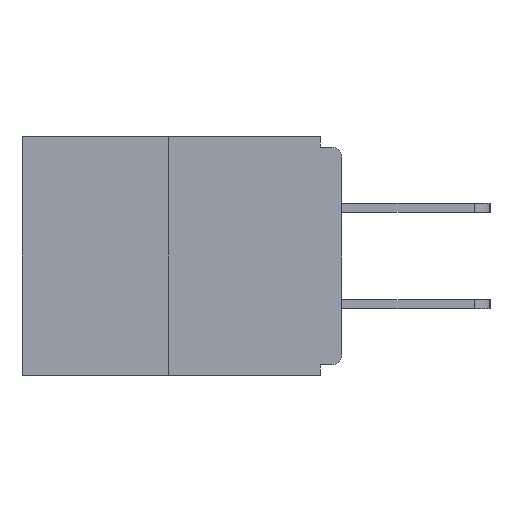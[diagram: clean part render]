
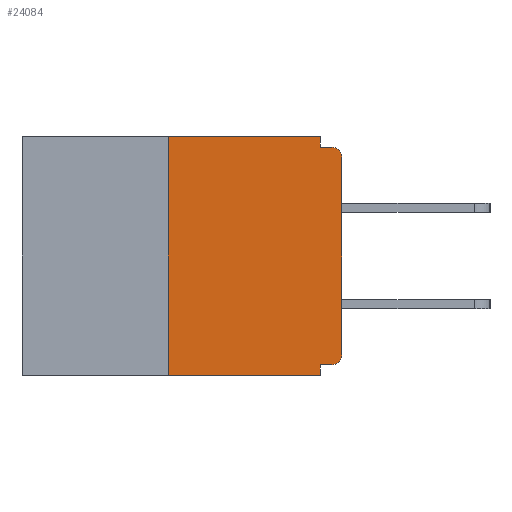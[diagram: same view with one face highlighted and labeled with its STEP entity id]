
A CAD part, left-side view. The second image highlights one B-rep face of the part: STEP entity #24084.
In plain terms, the highlighted planar face has unit normal (-1, 0, 0).
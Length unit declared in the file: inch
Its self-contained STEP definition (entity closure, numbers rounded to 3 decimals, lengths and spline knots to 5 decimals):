
#479 = CARTESIAN_POINT ( 'NONE',  ( 0., 0., -0.015 ) ) ;
#733 = ORIENTED_EDGE ( 'NONE', *, *, #24782, .F. ) ;
#1208 = VERTEX_POINT ( 'NONE', #2140 ) ;
#2140 = CARTESIAN_POINT ( 'NONE',  ( 0., 0.25, -0.343 ) ) ;
#2217 = VERTEX_POINT ( 'NONE', #22317 ) ;
#2232 = CARTESIAN_POINT ( 'NONE',  ( 0., 0., 0. ) ) ;
#2408 = DIRECTION ( 'NONE',  ( 0., 0., -1. ) ) ;
#2773 = CARTESIAN_POINT ( 'NONE',  ( 0., 0.46, 0. ) ) ;
#3001 = DIRECTION ( 'NONE',  ( 0., -1., 0. ) ) ;
#3303 = EDGE_CURVE ( 'NONE', #14553, #17531, #26968, .T. ) ;
#3306 = VERTEX_POINT ( 'NONE', #26632 ) ;
#3439 = VECTOR ( 'NONE', #9240, 39.37008 ) ;
#4180 = AXIS2_PLACEMENT_3D ( 'NONE', #10762, #8882, #2408 ) ;
#5092 = DIRECTION ( 'NONE',  ( 0., -1., 0. ) ) ;
#5288 = CARTESIAN_POINT ( 'NONE',  ( 0., 0., -0.03 ) ) ;
#5562 = ORIENTED_EDGE ( 'NONE', *, *, #7848, .T. ) ;
#6050 = ORIENTED_EDGE ( 'NONE', *, *, #3303, .T. ) ;
#6317 = ORIENTED_EDGE ( 'NONE', *, *, #28111, .F. ) ;
#7618 = LINE ( 'NONE', #24340, #26913 ) ;
#7848 = EDGE_CURVE ( 'NONE', #1208, #15797, #12713, .T. ) ;
#7966 = VERTEX_POINT ( 'NONE', #12307 ) ;
#8200 = DIRECTION ( 'NONE',  ( 0., 0., -1. ) ) ;
#8882 = DIRECTION ( 'NONE',  ( -1., 0., 0. ) ) ;
#9086 = DIRECTION ( 'NONE',  ( 0., 0., 1. ) ) ;
#9240 = DIRECTION ( 'NONE',  ( 0., 1., 0. ) ) ;
#9381 = LINE ( 'NONE', #25007, #3439 ) ;
#9680 = ORIENTED_EDGE ( 'NONE', *, *, #12728, .F. ) ;
#9987 = DIRECTION ( 'NONE',  ( 0., 0., 1. ) ) ;
#10334 = VERTEX_POINT ( 'NONE', #25268 ) ;
#10539 = AXIS2_PLACEMENT_3D ( 'NONE', #26731, #24196, #24578 ) ;
#10762 = CARTESIAN_POINT ( 'NONE',  ( 0., 0.015, -0.313 ) ) ;
#11080 = VERTEX_POINT ( 'NONE', #20988 ) ;
#11136 = VERTEX_POINT ( 'NONE', #15093 ) ;
#11830 = EDGE_CURVE ( 'NONE', #3306, #15797, #7618, .T. ) ;
#12169 = CARTESIAN_POINT ( 'NONE',  ( 0., 0.031, -0.343 ) ) ;
#12170 = VECTOR ( 'NONE', #14246, 39.37008 ) ;
#12307 = CARTESIAN_POINT ( 'NONE',  ( 0., 0.015, -0.328 ) ) ;
#12713 = LINE ( 'NONE', #25426, #21803 ) ;
#12716 = PLANE ( 'NONE',  #27837 ) ;
#12728 = EDGE_CURVE ( 'NONE', #11136, #17531, #20529, .T. ) ;
#13058 = ORIENTED_EDGE ( 'NONE', *, *, #28562, .F. ) ;
#14246 = DIRECTION ( 'NONE',  ( 0., -1., 0. ) ) ;
#14265 = EDGE_CURVE ( 'NONE', #10334, #14553, #19406, .T. ) ;
#14553 = VERTEX_POINT ( 'NONE', #5288 ) ;
#14580 = VECTOR ( 'NONE', #5092, 39.37008 ) ;
#14859 = CARTESIAN_POINT ( 'NONE',  ( 0., 0.031, 0. ) ) ;
#14951 = EDGE_CURVE ( 'NONE', #7966, #10334, #27060, .T. ) ;
#15093 = CARTESIAN_POINT ( 'NONE',  ( 0., 0.031, -0.015 ) ) ;
#15196 = EDGE_LOOP ( 'NONE', ( #13058, #733, #5562, #18835, #19710, #15767, #25383, #6050, #9680, #6317 ) ) ;
#15767 = ORIENTED_EDGE ( 'NONE', *, *, #14951, .T. ) ;
#15797 = VERTEX_POINT ( 'NONE', #12169 ) ;
#16951 = CARTESIAN_POINT ( 'NONE',  ( 0., 0.46, 0. ) ) ;
#17133 = DIRECTION ( 'NONE',  ( 0., 0., -1. ) ) ;
#17531 = VERTEX_POINT ( 'NONE', #27202 ) ;
#18835 = ORIENTED_EDGE ( 'NONE', *, *, #11830, .F. ) ;
#19326 = EDGE_CURVE ( 'NONE', #7966, #3306, #9381, .T. ) ;
#19406 = LINE ( 'NONE', #2232, #21489 ) ;
#19710 = ORIENTED_EDGE ( 'NONE', *, *, #19326, .F. ) ;
#20522 = VECTOR ( 'NONE', #9987, 39.37008 ) ;
#20529 = LINE ( 'NONE', #479, #14580 ) ;
#20988 = CARTESIAN_POINT ( 'NONE',  ( 0., 0.25, 0. ) ) ;
#21480 = LINE ( 'NONE', #14859, #27426 ) ;
#21489 = VECTOR ( 'NONE', #9086, 39.37008 ) ;
#21714 = DIRECTION ( 'NONE',  ( 1., 0., 0. ) ) ;
#21803 = VECTOR ( 'NONE', #3001, 39.37008 ) ;
#22317 = CARTESIAN_POINT ( 'NONE',  ( 0., 0.031, 0. ) ) ;
#22673 = LINE ( 'NONE', #2773, #12170 ) ;
#24084 = ADVANCED_FACE ( 'NONE', ( #26532 ), #12716, .F. ) ;
#24196 = DIRECTION ( 'NONE',  ( -1., 0., 0. ) ) ;
#24340 = CARTESIAN_POINT ( 'NONE',  ( 0., 0.031, -0.343 ) ) ;
#24578 = DIRECTION ( 'NONE',  ( 0., 0., -1. ) ) ;
#24782 = EDGE_CURVE ( 'NONE', #1208, #11080, #26470, .T. ) ;
#25007 = CARTESIAN_POINT ( 'NONE',  ( 0., 0., -0.328 ) ) ;
#25185 = CARTESIAN_POINT ( 'NONE',  ( 0., 0.25, 0. ) ) ;
#25268 = CARTESIAN_POINT ( 'NONE',  ( 0., 0., -0.313 ) ) ;
#25383 = ORIENTED_EDGE ( 'NONE', *, *, #14265, .T. ) ;
#25426 = CARTESIAN_POINT ( 'NONE',  ( 0., 0.46, -0.343 ) ) ;
#26470 = LINE ( 'NONE', #25185, #20522 ) ;
#26532 = FACE_OUTER_BOUND ( 'NONE', #15196, .T. ) ;
#26632 = CARTESIAN_POINT ( 'NONE',  ( 0., 0.031, -0.328 ) ) ;
#26681 = DIRECTION ( 'NONE',  ( 0., 0., -1. ) ) ;
#26731 = CARTESIAN_POINT ( 'NONE',  ( 0., 0.015, -0.03 ) ) ;
#26913 = VECTOR ( 'NONE', #26681, 39.37008 ) ;
#26968 = CIRCLE ( 'NONE', #10539, 0.015 ) ;
#27060 = CIRCLE ( 'NONE', #4180, 0.015 ) ;
#27202 = CARTESIAN_POINT ( 'NONE',  ( 0., 0.015, -0.015 ) ) ;
#27426 = VECTOR ( 'NONE', #17133, 39.37008 ) ;
#27837 = AXIS2_PLACEMENT_3D ( 'NONE', #16951, #21714, #8200 ) ;
#28111 = EDGE_CURVE ( 'NONE', #2217, #11136, #21480, .T. ) ;
#28562 = EDGE_CURVE ( 'NONE', #11080, #2217, #22673, .T. ) ;
